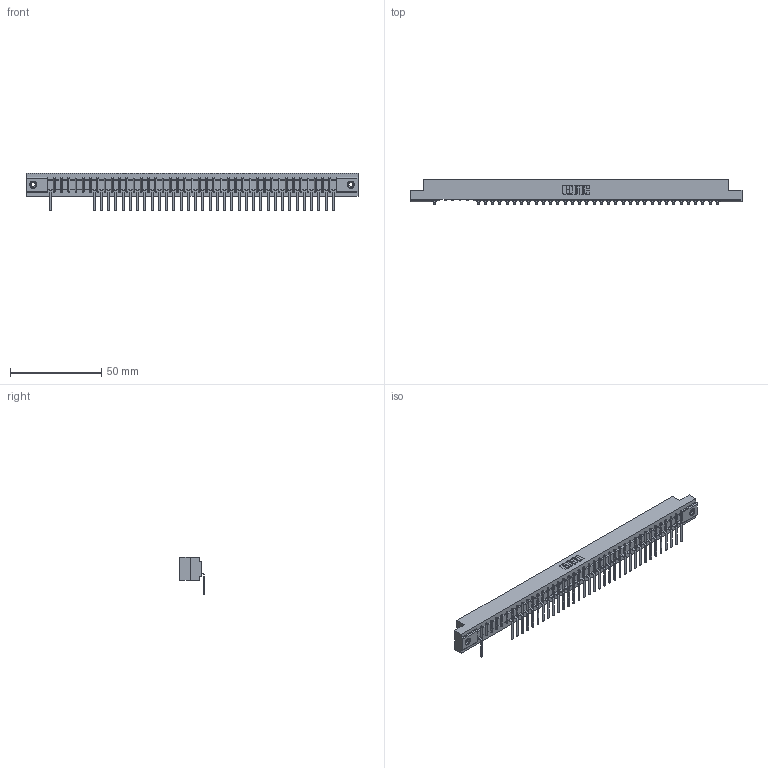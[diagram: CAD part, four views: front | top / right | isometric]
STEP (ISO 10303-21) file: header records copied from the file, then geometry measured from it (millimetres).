
FILE_DESCRIPTION (( 'STEP AP203' ), '1' );
FILE_NAME ('357-040-557-108.STEP', '2018-08-11T05:38:05', ( '' ), ( '' ), 'SwSTEP 2.0', 'SolidWorks 2016', '' );
FILE_SCHEMA (( 'CONFIG_CONTROL_DESIGN' ));
Length unit declared in the file: inch
Products named in the file (4): 307 Part_.156 Dia Mounting Holes; 307-290-002_557; 345-250-001_345-250-003-102; 357-040-557-108
Assembly tree (38 placements, depth 2):
  357-040-557-108
    307 Part_.156 Dia Mounting Holes
    307-290-002_557  x35
    345-250-001_345-250-003-102  x2
Bounding box: 181.51 x 13.32 x 20.66 mm (x, y, z)
Volume: 19352 mm3; surface area: 23995.4 mm2
Topology: 38 solids, 38 shells, 3049 faces, 9319 edges, 6094 vertices
Faces by surface type: plane 1807, cylinder 1144, sphere 82, cone 12, torus 4
Entity records: 36417 total; most frequent: CARTESIAN_POINT 6146, ORIENTED_EDGE 6134, DIRECTION 5977, EDGE_CURVE 3067, LINE 2347, VECTOR 2347, VERTEX_POINT 1984, AXIS2_PLACEMENT_3D 1815
